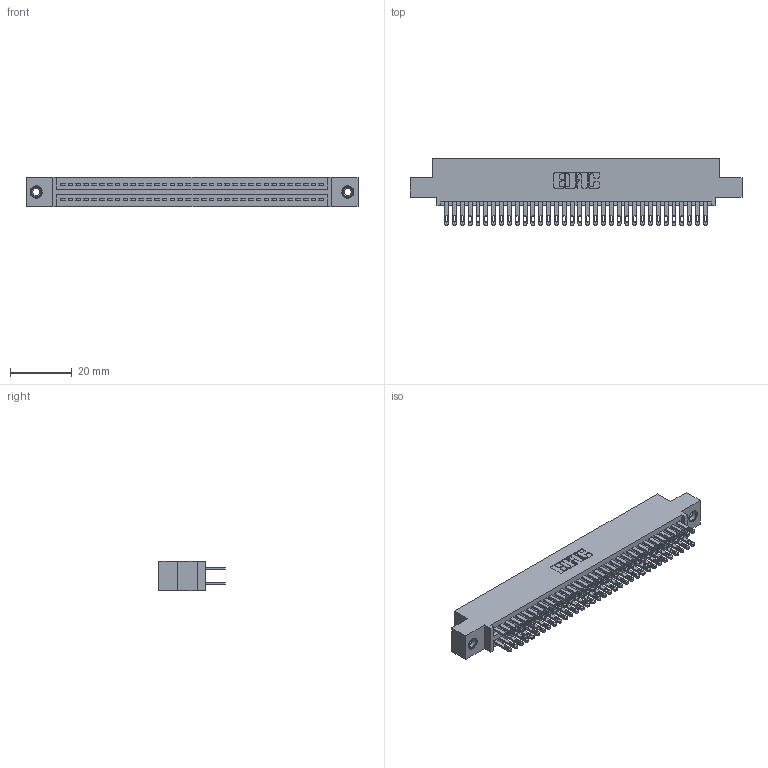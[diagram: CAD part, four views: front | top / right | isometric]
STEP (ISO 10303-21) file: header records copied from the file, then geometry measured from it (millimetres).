
FILE_DESCRIPTION (( 'STEP AP203' ), '1' );
FILE_NAME ('895-068-500-508.STEP', '2020-09-28T15:22:30', ( '' ), ( '' ), 'SwSTEP 2.0', 'SolidWorks 2020', '' );
FILE_SCHEMA (( 'CONFIG_CONTROL_DESIGN' ));
Length unit declared in the file: inch
Products named in the file (4): 845 Part_0.110 Offset - 0.156 Dia-TI; 895-068-500-508; 345-292-001_345-293-100; 345-250-001_345-250-003-102
Assembly tree (71 placements, depth 2):
  895-068-500-508
    845 Part_0.110 Offset - 0.156 Dia-TI
    345-292-001_345-293-100  x68
    345-250-001_345-250-003-102  x2
Bounding box: 107.57 x 21.51 x 9.4 mm (x, y, z)
Volume: 10503 mm3; surface area: 16170.1 mm2
Topology: 71 solids, 71 shells, 3318 faces, 10077 edges, 6710 vertices
Faces by surface type: plane 1952, cylinder 1350, cone 12, torus 4
Entity records: 29002 total; most frequent: CARTESIAN_POINT 4851, ORIENTED_EDGE 4778, DIRECTION 4315, EDGE_CURVE 2389, LINE 2097, VECTOR 2097, VERTEX_POINT 1588, AXIS2_PLACEMENT_3D 1109
